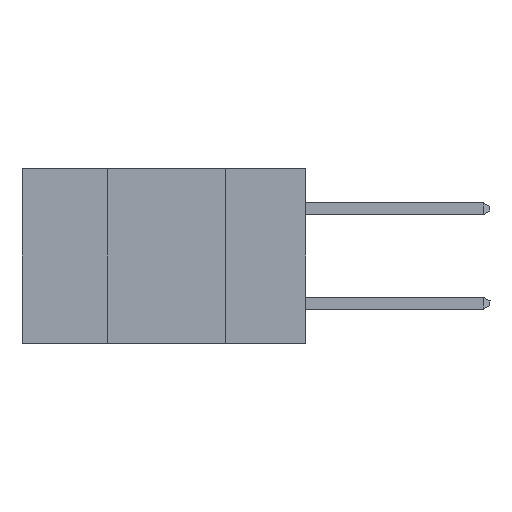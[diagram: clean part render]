
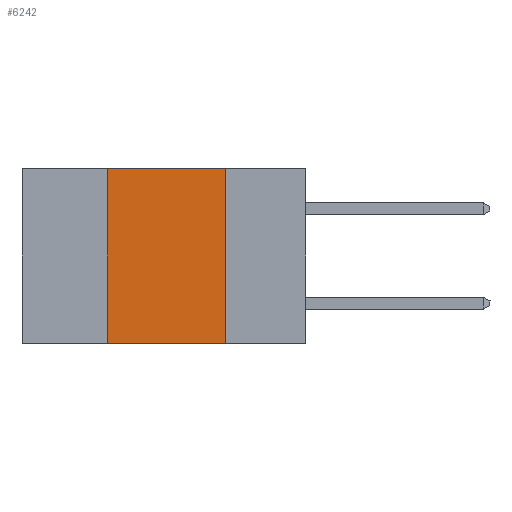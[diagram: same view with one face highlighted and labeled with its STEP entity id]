
A CAD part, left-side view. The second image highlights one B-rep face of the part: STEP entity #6242.
In plain terms, the highlighted planar face has unit normal (-1, 0, 0).
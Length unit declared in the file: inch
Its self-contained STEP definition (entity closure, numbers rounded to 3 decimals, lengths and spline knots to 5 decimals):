
#26 = FACE_OUTER_BOUND ( 'NONE', #5313, .T. ) ;
#381 = DIRECTION ( 'NONE',  ( 0., 0., -1. ) ) ;
#565 = ORIENTED_EDGE ( 'NONE', *, *, #2615, .F. ) ;
#1592 = VECTOR ( 'NONE', #4191, 39.37008 ) ;
#1898 = CARTESIAN_POINT ( 'NONE',  ( 0., 0.17, 0. ) ) ;
#2358 = CARTESIAN_POINT ( 'NONE',  ( 0., 0.17, 0. ) ) ;
#2615 = EDGE_CURVE ( 'NONE', #9541, #4427, #8081, .T. ) ;
#3000 = VECTOR ( 'NONE', #5282, 39.37008 ) ;
#3100 = CARTESIAN_POINT ( 'NONE',  ( 0., 0.42, 0. ) ) ;
#3210 = DIRECTION ( 'NONE',  ( 0., -1., 0. ) ) ;
#4118 = ORIENTED_EDGE ( 'NONE', *, *, #8458, .T. ) ;
#4191 = DIRECTION ( 'NONE',  ( 0., 0., 1. ) ) ;
#4427 = VERTEX_POINT ( 'NONE', #3100 ) ;
#4846 = AXIS2_PLACEMENT_3D ( 'NONE', #5197, #11995, #381 ) ;
#5197 = CARTESIAN_POINT ( 'NONE',  ( 0., 0.6, 0. ) ) ;
#5240 = CARTESIAN_POINT ( 'NONE',  ( 0., 0.6, -0.37 ) ) ;
#5257 = LINE ( 'NONE', #5240, #10138 ) ;
#5282 = DIRECTION ( 'NONE',  ( 0., -1., 0. ) ) ;
#5313 = EDGE_LOOP ( 'NONE', ( #9062, #5328, #565, #4118 ) ) ;
#5328 = ORIENTED_EDGE ( 'NONE', *, *, #8855, .F. ) ;
#5566 = CARTESIAN_POINT ( 'NONE',  ( 0., 0.42, -0.37 ) ) ;
#6242 = ADVANCED_FACE ( 'NONE', ( #26 ), #9077, .F. ) ;
#6464 = VERTEX_POINT ( 'NONE', #6945 ) ;
#6945 = CARTESIAN_POINT ( 'NONE',  ( 0., 0.17, -0.37 ) ) ;
#7224 = CARTESIAN_POINT ( 'NONE',  ( 0., 0.6, 0. ) ) ;
#7511 = LINE ( 'NONE', #2358, #10564 ) ;
#8081 = LINE ( 'NONE', #11859, #1592 ) ;
#8128 = LINE ( 'NONE', #7224, #3000 ) ;
#8458 = EDGE_CURVE ( 'NONE', #9541, #6464, #5257, .T. ) ;
#8855 = EDGE_CURVE ( 'NONE', #4427, #11157, #8128, .T. ) ;
#9058 = EDGE_CURVE ( 'NONE', #11157, #6464, #7511, .T. ) ;
#9062 = ORIENTED_EDGE ( 'NONE', *, *, #9058, .F. ) ;
#9077 = PLANE ( 'NONE',  #4846 ) ;
#9541 = VERTEX_POINT ( 'NONE', #5566 ) ;
#10138 = VECTOR ( 'NONE', #3210, 39.37008 ) ;
#10564 = VECTOR ( 'NONE', #11730, 39.37008 ) ;
#11157 = VERTEX_POINT ( 'NONE', #1898 ) ;
#11730 = DIRECTION ( 'NONE',  ( 0., 0., -1. ) ) ;
#11859 = CARTESIAN_POINT ( 'NONE',  ( 0., 0.42, 0. ) ) ;
#11995 = DIRECTION ( 'NONE',  ( 1., 0., 0. ) ) ;
